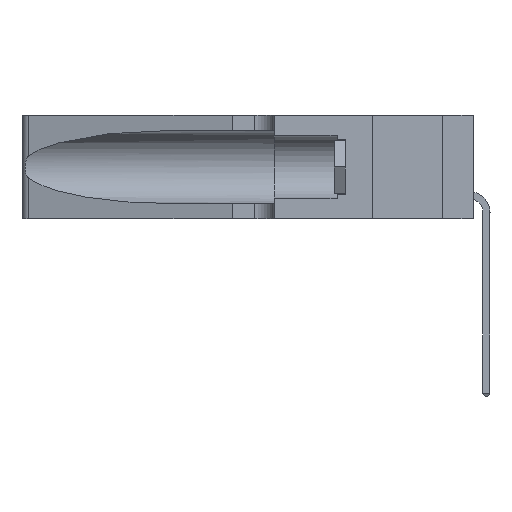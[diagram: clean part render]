
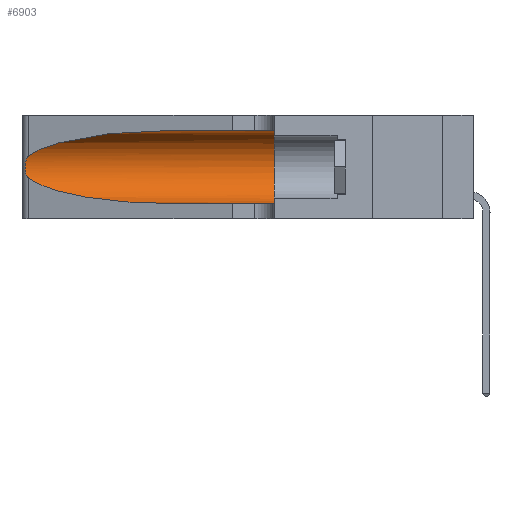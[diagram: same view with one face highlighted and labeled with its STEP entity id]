
A CAD part, left-side view. The second image highlights one B-rep face of the part: STEP entity #6903.
In plain terms, the highlighted cylindrical face has radius 3.308 mm (diameter 6.617 mm), a partial arc.
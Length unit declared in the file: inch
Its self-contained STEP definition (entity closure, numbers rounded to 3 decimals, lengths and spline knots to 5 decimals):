
#104 = CARTESIAN_POINT ( 'NONE',  ( 0.25487, 1.22718, 0.22369 ) ) ;
#390 =( BOUNDED_CURVE ( )  B_SPLINE_CURVE ( 3, ( #29256, #2339, #9815, #22540 ),
 .UNSPECIFIED., .F., .F. ) 
 B_SPLINE_CURVE_WITH_KNOTS ( ( 4, 4 ),
 ( 1.5708, 2.84003 ),
 .UNSPECIFIED. ) 
 CURVE ( )  GEOMETRIC_REPRESENTATION_ITEM ( )  RATIONAL_B_SPLINE_CURVE ( ( 1., 0.87, 0.87, 1. ) ) 
 REPRESENTATION_ITEM ( '' )  );
#550 = VERTEX_POINT ( 'NONE', #4113 ) ;
#1482 = EDGE_CURVE ( 'NONE', #15838, #550, #18857, .T. ) ;
#1806 = EDGE_CURVE ( 'NONE', #18983, #2816, #390, .T. ) ;
#2339 = CARTESIAN_POINT ( 'NONE',  ( 0.18966, 0.96281, 0.31525 ) ) ;
#2719 = CARTESIAN_POINT ( 'NONE',  ( 0.25555, 1.22993, 0.14849 ) ) ;
#2816 = VERTEX_POINT ( 'NONE', #21900 ) ;
#3133 = EDGE_CURVE ( 'NONE', #18983, #7396, #7017, .T. ) ;
#4113 = CARTESIAN_POINT ( 'NONE',  ( 0.1305, 0.35, 0.05475 ) ) ;
#4260 = CARTESIAN_POINT ( 'NONE',  ( 0.1305, 0.35, 0.31525 ) ) ;
#5096 = CARTESIAN_POINT ( 'NONE',  ( 0.25854, 1.2359, 0.20912 ) ) ;
#6184 =( BOUNDED_CURVE ( )  B_SPLINE_CURVE ( 3, ( #20453, #18199, #8146, #15810 ),
 .UNSPECIFIED., .F., .T. ) 
 B_SPLINE_CURVE_WITH_KNOTS ( ( 4, 4 ),
 ( 3.44316, 4.71239 ),
 .UNSPECIFIED. ) 
 CURVE ( )  GEOMETRIC_REPRESENTATION_ITEM ( )  RATIONAL_B_SPLINE_CURVE ( ( 1., 0.87, 0.87, 1. ) ) 
 REPRESENTATION_ITEM ( '' )  );
#6195 = EDGE_CURVE ( 'NONE', #16581, #15838, #6184, .T. ) ;
#6754 = VECTOR ( 'NONE', #7340, 39.37008 ) ;
#6903 = ADVANCED_FACE ( 'NONE', ( #32058 ), #28189, .F. ) ;
#7017 = LINE ( 'NONE', #31228, #29942 ) ;
#7340 = DIRECTION ( 'NONE',  ( 0., -1., 0. ) ) ;
#7396 = VERTEX_POINT ( 'NONE', #4260 ) ;
#8146 = CARTESIAN_POINT ( 'NONE',  ( 0.18966, 0.96281, 0.05475 ) ) ;
#9801 = EDGE_CURVE ( 'NONE', #7396, #550, #31196, .T. ) ;
#9815 = CARTESIAN_POINT ( 'NONE',  ( 0.2373, 1.15595, 0.28018 ) ) ;
#10105 = CARTESIAN_POINT ( 'NONE',  ( 0.26018, 1.23835, 0.19895 ) ) ;
#10313 = CARTESIAN_POINT ( 'NONE',  ( 0.25639, 1.23186, 0.15144 ) ) ;
#10359 = EDGE_LOOP ( 'NONE', ( #31575, #21512, #24780, #20141, #24806, #16307 ) ) ;
#11375 = B_SPLINE_CURVE_WITH_KNOTS ( 'NONE', 3,
 ( #104, #17540, #30063, #20021, #5096, #10105, #27789, #12845, #25197, #22515, #17746, #10313, #2719, #29757 ),
 .UNSPECIFIED., .F., .F.,
 ( 4, 2, 2, 2, 2, 2, 4 ),
 ( 0., 0.00027, 0.00053, 0.00107, 0.0016, 0.00187, 0.00214 ),
 .UNSPECIFIED. ) ;
#11515 = DIRECTION ( 'NONE',  ( 0., -1., 0. ) ) ;
#12174 = CARTESIAN_POINT ( 'NONE',  ( 0.1305, 0.72297, 0.05475 ) ) ;
#12363 = CARTESIAN_POINT ( 'NONE',  ( 0.1305, 1.61858, 0.05475 ) ) ;
#12406 = DIRECTION ( 'NONE',  ( 0., -1., 0. ) ) ;
#12845 = CARTESIAN_POINT ( 'NONE',  ( 0.26075, 1.23896, 0.178 ) ) ;
#14664 = AXIS2_PLACEMENT_3D ( 'NONE', #24468, #12406, #22404 ) ;
#15810 = CARTESIAN_POINT ( 'NONE',  ( 0.1305, 0.72297, 0.05475 ) ) ;
#15838 = VERTEX_POINT ( 'NONE', #12174 ) ;
#16307 = ORIENTED_EDGE ( 'NONE', *, *, #3133, .F. ) ;
#16581 = VERTEX_POINT ( 'NONE', #25405 ) ;
#17014 = AXIS2_PLACEMENT_3D ( 'NONE', #23808, #23912, #17365 ) ;
#17365 = DIRECTION ( 'NONE',  ( 0., 0., 1. ) ) ;
#17540 = CARTESIAN_POINT ( 'NONE',  ( 0.25555, 1.22994, 0.2215 ) ) ;
#17746 = CARTESIAN_POINT ( 'NONE',  ( 0.25789, 1.23486, 0.15765 ) ) ;
#18199 = CARTESIAN_POINT ( 'NONE',  ( 0.2373, 1.15595, 0.08982 ) ) ;
#18857 = LINE ( 'NONE', #12363, #6754 ) ;
#18983 = VERTEX_POINT ( 'NONE', #20854 ) ;
#20021 = CARTESIAN_POINT ( 'NONE',  ( 0.25787, 1.23484, 0.2124 ) ) ;
#20141 = ORIENTED_EDGE ( 'NONE', *, *, #1482, .T. ) ;
#20453 = CARTESIAN_POINT ( 'NONE',  ( 0.25487, 1.22718, 0.14631 ) ) ;
#20854 = CARTESIAN_POINT ( 'NONE',  ( 0.1305, 0.72297, 0.31525 ) ) ;
#21512 = ORIENTED_EDGE ( 'NONE', *, *, #28622, .T. ) ;
#21900 = CARTESIAN_POINT ( 'NONE',  ( 0.25487, 1.22718, 0.22369 ) ) ;
#22404 = DIRECTION ( 'NONE',  ( 0., 0., -1. ) ) ;
#22515 = CARTESIAN_POINT ( 'NONE',  ( 0.25856, 1.23593, 0.16098 ) ) ;
#22540 = CARTESIAN_POINT ( 'NONE',  ( 0.25487, 1.22718, 0.22369 ) ) ;
#23808 = CARTESIAN_POINT ( 'NONE',  ( 0.1305, 0.35, 0.185 ) ) ;
#23912 = DIRECTION ( 'NONE',  ( 0., 1., 0. ) ) ;
#24468 = CARTESIAN_POINT ( 'NONE',  ( 0.1305, 1.61858, 0.185 ) ) ;
#24780 = ORIENTED_EDGE ( 'NONE', *, *, #6195, .T. ) ;
#24806 = ORIENTED_EDGE ( 'NONE', *, *, #9801, .F. ) ;
#25197 = CARTESIAN_POINT ( 'NONE',  ( 0.26017, 1.23833, 0.17102 ) ) ;
#25405 = CARTESIAN_POINT ( 'NONE',  ( 0.25487, 1.22718, 0.14631 ) ) ;
#27789 = CARTESIAN_POINT ( 'NONE',  ( 0.26075, 1.23896, 0.19203 ) ) ;
#28189 = CYLINDRICAL_SURFACE ( 'NONE', #14664, 0.13025 ) ;
#28622 = EDGE_CURVE ( 'NONE', #2816, #16581, #11375, .T. ) ;
#29256 = CARTESIAN_POINT ( 'NONE',  ( 0.1305, 0.72297, 0.31525 ) ) ;
#29757 = CARTESIAN_POINT ( 'NONE',  ( 0.25487, 1.22718, 0.14631 ) ) ;
#29942 = VECTOR ( 'NONE', #11515, 39.37008 ) ;
#30063 = CARTESIAN_POINT ( 'NONE',  ( 0.25639, 1.23184, 0.21858 ) ) ;
#31196 = CIRCLE ( 'NONE', #17014, 0.13025 ) ;
#31228 = CARTESIAN_POINT ( 'NONE',  ( 0.1305, 1.61858, 0.31525 ) ) ;
#31575 = ORIENTED_EDGE ( 'NONE', *, *, #1806, .T. ) ;
#32058 = FACE_OUTER_BOUND ( 'NONE', #10359, .T. ) ;
